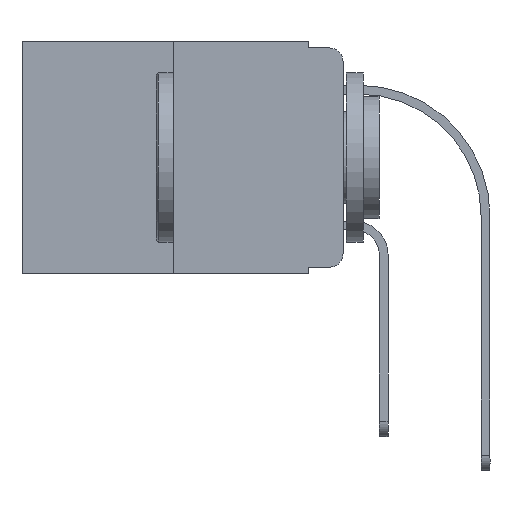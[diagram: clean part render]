
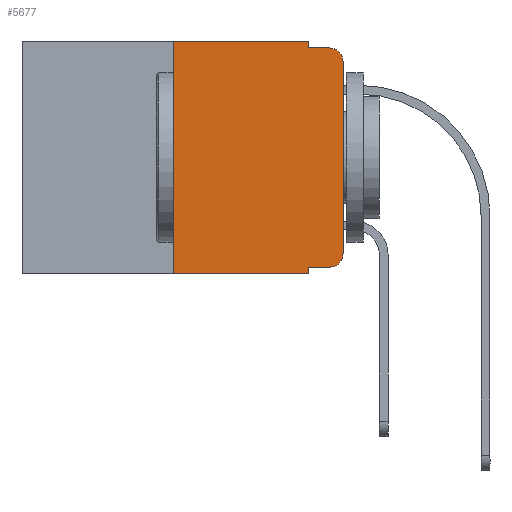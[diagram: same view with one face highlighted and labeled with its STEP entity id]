
A CAD part, left-side view. The second image highlights one B-rep face of the part: STEP entity #5677.
In plain terms, the highlighted planar face has unit normal (-1, 0, 0).
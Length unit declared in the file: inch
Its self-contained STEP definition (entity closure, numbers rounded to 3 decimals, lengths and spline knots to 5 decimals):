
#51 = CARTESIAN_POINT ( 'NONE',  ( 0., 0.051, -0.01 ) ) ;
#144 = VECTOR ( 'NONE', #9341, 39.37008 ) ;
#239 = EDGE_CURVE ( 'NONE', #11090, #11336, #4737, .T. ) ;
#285 = CARTESIAN_POINT ( 'NONE',  ( 0., 0.02, -0.313 ) ) ;
#323 = ORIENTED_EDGE ( 'NONE', *, *, #488, .T. ) ;
#342 = DIRECTION ( 'NONE',  ( -1., 0., 0. ) ) ;
#488 = EDGE_CURVE ( 'NONE', #4474, #6280, #5461, .T. ) ;
#568 = DIRECTION ( 'NONE',  ( 0., 0., -1. ) ) ;
#668 = ORIENTED_EDGE ( 'NONE', *, *, #11683, .T. ) ;
#822 = DIRECTION ( 'NONE',  ( 0., -1., 0. ) ) ;
#954 = LINE ( 'NONE', #1768, #4755 ) ;
#1312 = DIRECTION ( 'NONE',  ( 1., 0., 0. ) ) ;
#1397 = AXIS2_PLACEMENT_3D ( 'NONE', #8661, #5618, #6670 ) ;
#1594 = ORIENTED_EDGE ( 'NONE', *, *, #239, .T. ) ;
#1768 = CARTESIAN_POINT ( 'NONE',  ( 0., 0., 0. ) ) ;
#1804 = CARTESIAN_POINT ( 'NONE',  ( 0., 0.25, -0.343 ) ) ;
#2117 = CARTESIAN_POINT ( 'NONE',  ( 0., 0.473, 0. ) ) ;
#2138 = VERTEX_POINT ( 'NONE', #10770 ) ;
#2246 = CARTESIAN_POINT ( 'NONE',  ( 0., 0.473, 0. ) ) ;
#2307 = DIRECTION ( 'NONE',  ( 0., 0., 1. ) ) ;
#2385 = AXIS2_PLACEMENT_3D ( 'NONE', #285, #342, #3943 ) ;
#2804 = EDGE_CURVE ( 'NONE', #9924, #7111, #7749, .T. ) ;
#2830 = ORIENTED_EDGE ( 'NONE', *, *, #9854, .F. ) ;
#3034 = CARTESIAN_POINT ( 'NONE',  ( 0., 0.473, -0.343 ) ) ;
#3172 = CARTESIAN_POINT ( 'NONE',  ( 0., 0.25, 0. ) ) ;
#3387 = CARTESIAN_POINT ( 'NONE',  ( 0., 0.051, 0. ) ) ;
#3915 = DIRECTION ( 'NONE',  ( 0., -1., 0. ) ) ;
#3923 = ORIENTED_EDGE ( 'NONE', *, *, #7178, .F. ) ;
#3943 = DIRECTION ( 'NONE',  ( 0., 0., -1. ) ) ;
#4474 = VERTEX_POINT ( 'NONE', #6334 ) ;
#4737 = LINE ( 'NONE', #3034, #10094 ) ;
#4755 = VECTOR ( 'NONE', #7431, 39.37008 ) ;
#4908 = AXIS2_PLACEMENT_3D ( 'NONE', #2246, #1312, #568 ) ;
#5461 = LINE ( 'NONE', #11080, #10111 ) ;
#5618 = DIRECTION ( 'NONE',  ( -1., 0., 0. ) ) ;
#5642 = EDGE_CURVE ( 'NONE', #8933, #2138, #5917, .T. ) ;
#5661 = DIRECTION ( 'NONE',  ( 0., 0., -1. ) ) ;
#5677 = ADVANCED_FACE ( 'NONE', ( #6973 ), #10780, .F. ) ;
#5681 = CARTESIAN_POINT ( 'NONE',  ( 0., 0.25, 0. ) ) ;
#5900 = CARTESIAN_POINT ( 'NONE',  ( 0., 0.051, -0.343 ) ) ;
#5906 = VECTOR ( 'NONE', #7130, 39.37008 ) ;
#5917 = LINE ( 'NONE', #2117, #6299 ) ;
#5964 = EDGE_CURVE ( 'NONE', #4474, #11336, #7878, .T. ) ;
#5983 = LINE ( 'NONE', #3172, #12103 ) ;
#6280 = VERTEX_POINT ( 'NONE', #11477 ) ;
#6299 = VECTOR ( 'NONE', #3915, 39.37008 ) ;
#6334 = CARTESIAN_POINT ( 'NONE',  ( 0., 0.051, -0.333 ) ) ;
#6670 = DIRECTION ( 'NONE',  ( 0., 0., -1. ) ) ;
#6973 = FACE_OUTER_BOUND ( 'NONE', #11198, .T. ) ;
#7111 = VERTEX_POINT ( 'NONE', #9347 ) ;
#7130 = DIRECTION ( 'NONE',  ( 0., 0., -1. ) ) ;
#7178 = EDGE_CURVE ( 'NONE', #2138, #9843, #10274, .T. ) ;
#7204 = VECTOR ( 'NONE', #5661, 39.37008 ) ;
#7342 = CARTESIAN_POINT ( 'NONE',  ( 0., 0., -0.313 ) ) ;
#7431 = DIRECTION ( 'NONE',  ( 0., 0., 1. ) ) ;
#7749 = CIRCLE ( 'NONE', #1397, 0.02 ) ;
#7878 = LINE ( 'NONE', #3387, #5906 ) ;
#8060 = ORIENTED_EDGE ( 'NONE', *, *, #10902, .F. ) ;
#8326 = DIRECTION ( 'NONE',  ( 0., -1., 0. ) ) ;
#8525 = ORIENTED_EDGE ( 'NONE', *, *, #5642, .F. ) ;
#8661 = CARTESIAN_POINT ( 'NONE',  ( 0., 0.02, -0.03 ) ) ;
#8933 = VERTEX_POINT ( 'NONE', #5681 ) ;
#9126 = ORIENTED_EDGE ( 'NONE', *, *, #5964, .F. ) ;
#9136 = CIRCLE ( 'NONE', #2385, 0.02 ) ;
#9341 = DIRECTION ( 'NONE',  ( 0., -1., 0. ) ) ;
#9347 = CARTESIAN_POINT ( 'NONE',  ( 0., 0.02, -0.01 ) ) ;
#9576 = LINE ( 'NONE', #11446, #144 ) ;
#9620 = VERTEX_POINT ( 'NONE', #7342 ) ;
#9843 = VERTEX_POINT ( 'NONE', #51 ) ;
#9854 = EDGE_CURVE ( 'NONE', #9843, #7111, #9576, .T. ) ;
#9924 = VERTEX_POINT ( 'NONE', #10453 ) ;
#10021 = ORIENTED_EDGE ( 'NONE', *, *, #12048, .T. ) ;
#10094 = VECTOR ( 'NONE', #822, 39.37008 ) ;
#10111 = VECTOR ( 'NONE', #8326, 39.37008 ) ;
#10274 = LINE ( 'NONE', #10520, #7204 ) ;
#10453 = CARTESIAN_POINT ( 'NONE',  ( 0., 0., -0.03 ) ) ;
#10520 = CARTESIAN_POINT ( 'NONE',  ( 0., 0.051, 0. ) ) ;
#10770 = CARTESIAN_POINT ( 'NONE',  ( 0., 0.051, 0. ) ) ;
#10780 = PLANE ( 'NONE',  #4908 ) ;
#10902 = EDGE_CURVE ( 'NONE', #11090, #8933, #5983, .T. ) ;
#11080 = CARTESIAN_POINT ( 'NONE',  ( 0., 0.051, -0.333 ) ) ;
#11090 = VERTEX_POINT ( 'NONE', #1804 ) ;
#11198 = EDGE_LOOP ( 'NONE', ( #10021, #11722, #2830, #3923, #8525, #8060, #1594, #9126, #323, #668 ) ) ;
#11336 = VERTEX_POINT ( 'NONE', #5900 ) ;
#11446 = CARTESIAN_POINT ( 'NONE',  ( 0., 0.051, -0.01 ) ) ;
#11477 = CARTESIAN_POINT ( 'NONE',  ( 0., 0.02, -0.333 ) ) ;
#11683 = EDGE_CURVE ( 'NONE', #6280, #9620, #9136, .T. ) ;
#11722 = ORIENTED_EDGE ( 'NONE', *, *, #2804, .T. ) ;
#12048 = EDGE_CURVE ( 'NONE', #9620, #9924, #954, .T. ) ;
#12103 = VECTOR ( 'NONE', #2307, 39.37008 ) ;
